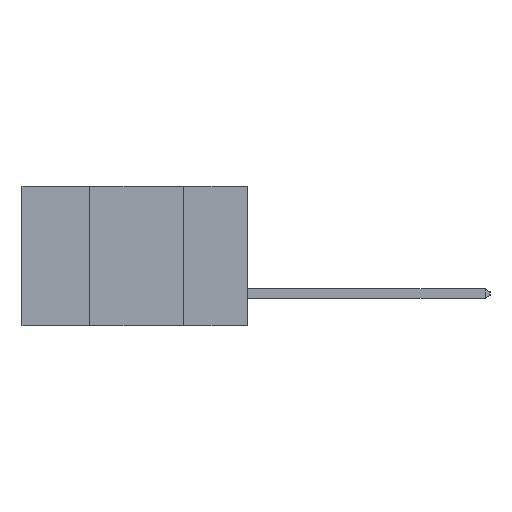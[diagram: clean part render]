
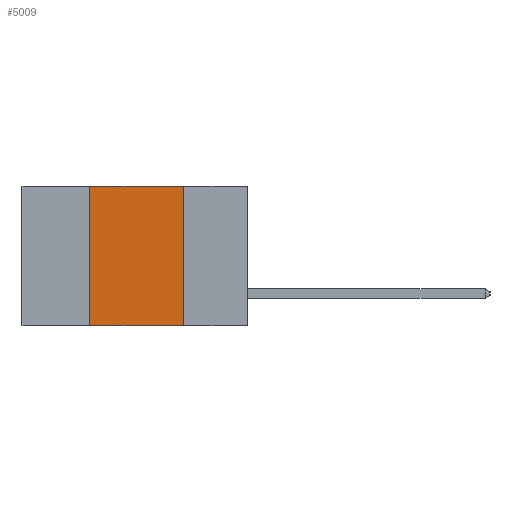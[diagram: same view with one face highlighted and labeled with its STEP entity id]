
A CAD part, left-side view. The second image highlights one B-rep face of the part: STEP entity #5009.
In plain terms, the highlighted planar face has unit normal (-1, 0, 0).
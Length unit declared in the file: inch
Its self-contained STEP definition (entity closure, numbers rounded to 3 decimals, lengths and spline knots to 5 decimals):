
#94 = ORIENTED_EDGE ( 'NONE', *, *, #875, .F. ) ;
#246 = CARTESIAN_POINT ( 'NONE',  ( 0., 0.17, -0.37 ) ) ;
#875 = EDGE_CURVE ( 'NONE', #2466, #5716, #6479, .T. ) ;
#1620 = DIRECTION ( 'NONE',  ( 0., 0., -1. ) ) ;
#1644 = CARTESIAN_POINT ( 'NONE',  ( 0., 0.17, 0. ) ) ;
#1690 = VECTOR ( 'NONE', #1620, 39.37008 ) ;
#1864 = LINE ( 'NONE', #2632, #10084 ) ;
#1993 = VERTEX_POINT ( 'NONE', #246 ) ;
#2274 = DIRECTION ( 'NONE',  ( 0., 0., -1. ) ) ;
#2466 = VERTEX_POINT ( 'NONE', #3529 ) ;
#2632 = CARTESIAN_POINT ( 'NONE',  ( 0., 0.6, 0. ) ) ;
#3400 = DIRECTION ( 'NONE',  ( 0., -1., 0. ) ) ;
#3529 = CARTESIAN_POINT ( 'NONE',  ( 0., 0.42, -0.37 ) ) ;
#3711 = DIRECTION ( 'NONE',  ( 0., 0., 1. ) ) ;
#3795 = CARTESIAN_POINT ( 'NONE',  ( 0., 0.42, 0. ) ) ;
#3803 = AXIS2_PLACEMENT_3D ( 'NONE', #10181, #9528, #2274 ) ;
#3863 = CARTESIAN_POINT ( 'NONE',  ( 0., 0.42, 0. ) ) ;
#4358 = VECTOR ( 'NONE', #3711, 39.37008 ) ;
#4651 = VERTEX_POINT ( 'NONE', #8895 ) ;
#4981 = LINE ( 'NONE', #7356, #8953 ) ;
#5009 = ADVANCED_FACE ( 'NONE', ( #8218 ), #9854, .F. ) ;
#5716 = VERTEX_POINT ( 'NONE', #3863 ) ;
#6229 = EDGE_CURVE ( 'NONE', #5716, #4651, #1864, .T. ) ;
#6251 = ORIENTED_EDGE ( 'NONE', *, *, #6229, .F. ) ;
#6479 = LINE ( 'NONE', #3795, #4358 ) ;
#7336 = EDGE_LOOP ( 'NONE', ( #8823, #6251, #94, #8070 ) ) ;
#7356 = CARTESIAN_POINT ( 'NONE',  ( 0., 0.6, -0.37 ) ) ;
#7378 = LINE ( 'NONE', #1644, #1690 ) ;
#7780 = EDGE_CURVE ( 'NONE', #4651, #1993, #7378, .T. ) ;
#8070 = ORIENTED_EDGE ( 'NONE', *, *, #10171, .T. ) ;
#8218 = FACE_OUTER_BOUND ( 'NONE', #7336, .T. ) ;
#8823 = ORIENTED_EDGE ( 'NONE', *, *, #7780, .F. ) ;
#8895 = CARTESIAN_POINT ( 'NONE',  ( 0., 0.17, 0. ) ) ;
#8953 = VECTOR ( 'NONE', #3400, 39.37008 ) ;
#9274 = DIRECTION ( 'NONE',  ( 0., -1., 0. ) ) ;
#9528 = DIRECTION ( 'NONE',  ( 1., 0., 0. ) ) ;
#9854 = PLANE ( 'NONE',  #3803 ) ;
#10084 = VECTOR ( 'NONE', #9274, 39.37008 ) ;
#10171 = EDGE_CURVE ( 'NONE', #2466, #1993, #4981, .T. ) ;
#10181 = CARTESIAN_POINT ( 'NONE',  ( 0., 0.6, 0. ) ) ;
